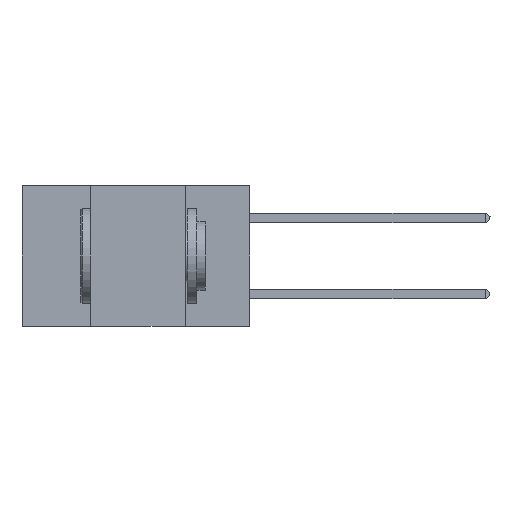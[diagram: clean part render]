
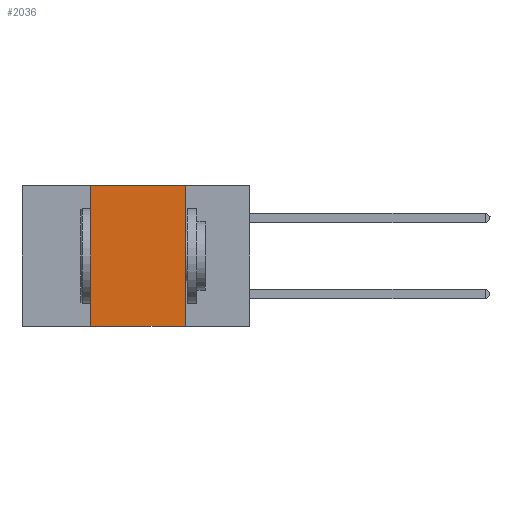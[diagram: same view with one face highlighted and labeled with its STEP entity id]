
A CAD part, left-side view. The second image highlights one B-rep face of the part: STEP entity #2036.
In plain terms, the highlighted planar face has unit normal (-1, 0, 0).
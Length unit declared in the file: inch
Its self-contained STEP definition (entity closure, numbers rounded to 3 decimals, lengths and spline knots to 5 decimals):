
#179 = ORIENTED_EDGE ( 'NONE', *, *, #6105, .F. ) ;
#359 = VECTOR ( 'NONE', #5495, 39.37008 ) ;
#395 = DIRECTION ( 'NONE',  ( 0., -1., 0. ) ) ;
#804 = VERTEX_POINT ( 'NONE', #9567 ) ;
#887 = LINE ( 'NONE', #6816, #3990 ) ;
#2036 = ADVANCED_FACE ( 'NONE', ( #8550 ), #4848, .F. ) ;
#2076 = VERTEX_POINT ( 'NONE', #5731 ) ;
#2578 = CARTESIAN_POINT ( 'NONE',  ( 0., 0.42, -0.37 ) ) ;
#3170 = VERTEX_POINT ( 'NONE', #8461 ) ;
#3392 = EDGE_CURVE ( 'NONE', #9651, #804, #887, .T. ) ;
#3561 = LINE ( 'NONE', #4382, #7975 ) ;
#3990 = VECTOR ( 'NONE', #395, 39.37008 ) ;
#4027 = CARTESIAN_POINT ( 'NONE',  ( 0., 0.42, 0. ) ) ;
#4382 = CARTESIAN_POINT ( 'NONE',  ( 0., 0.17, 0. ) ) ;
#4421 = VECTOR ( 'NONE', #5497, 39.37008 ) ;
#4848 = PLANE ( 'NONE',  #7705 ) ;
#5309 = EDGE_CURVE ( 'NONE', #9651, #2076, #9756, .T. ) ;
#5495 = DIRECTION ( 'NONE',  ( 0., 0., 1. ) ) ;
#5497 = DIRECTION ( 'NONE',  ( 0., -1., 0. ) ) ;
#5731 = CARTESIAN_POINT ( 'NONE',  ( 0., 0.42, 0. ) ) ;
#6105 = EDGE_CURVE ( 'NONE', #3170, #804, #3561, .T. ) ;
#6186 = DIRECTION ( 'NONE',  ( 0., 0., -1. ) ) ;
#6438 = CARTESIAN_POINT ( 'NONE',  ( 0., 0.6, 0. ) ) ;
#6816 = CARTESIAN_POINT ( 'NONE',  ( 0., 0.6, -0.37 ) ) ;
#7087 = CARTESIAN_POINT ( 'NONE',  ( 0., 0.6, 0. ) ) ;
#7269 = DIRECTION ( 'NONE',  ( 0., 0., -1. ) ) ;
#7705 = AXIS2_PLACEMENT_3D ( 'NONE', #6438, #9676, #7269 ) ;
#7755 = EDGE_CURVE ( 'NONE', #2076, #3170, #8743, .T. ) ;
#7975 = VECTOR ( 'NONE', #6186, 39.37008 ) ;
#8086 = ORIENTED_EDGE ( 'NONE', *, *, #3392, .T. ) ;
#8461 = CARTESIAN_POINT ( 'NONE',  ( 0., 0.17, 0. ) ) ;
#8515 = ORIENTED_EDGE ( 'NONE', *, *, #5309, .F. ) ;
#8550 = FACE_OUTER_BOUND ( 'NONE', #8643, .T. ) ;
#8592 = ORIENTED_EDGE ( 'NONE', *, *, #7755, .F. ) ;
#8643 = EDGE_LOOP ( 'NONE', ( #179, #8592, #8515, #8086 ) ) ;
#8743 = LINE ( 'NONE', #7087, #4421 ) ;
#9567 = CARTESIAN_POINT ( 'NONE',  ( 0., 0.17, -0.37 ) ) ;
#9651 = VERTEX_POINT ( 'NONE', #2578 ) ;
#9676 = DIRECTION ( 'NONE',  ( 1., 0., 0. ) ) ;
#9756 = LINE ( 'NONE', #4027, #359 ) ;
